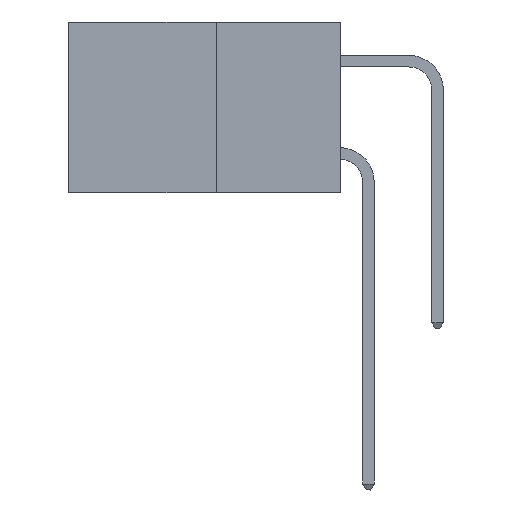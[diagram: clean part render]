
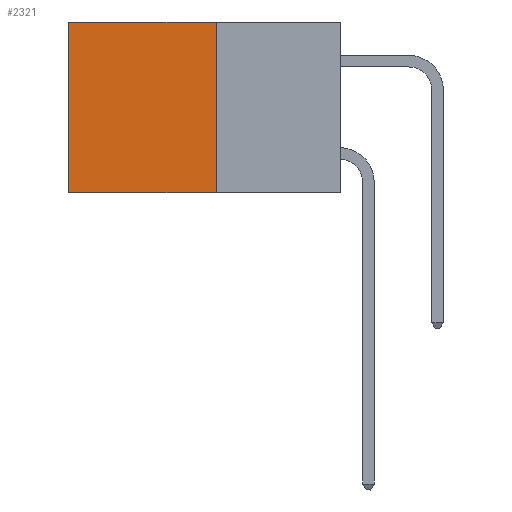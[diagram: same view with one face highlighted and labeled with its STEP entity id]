
A CAD part, left-side view. The second image highlights one B-rep face of the part: STEP entity #2321.
In plain terms, the highlighted planar face has unit normal (-1, 0, 0).
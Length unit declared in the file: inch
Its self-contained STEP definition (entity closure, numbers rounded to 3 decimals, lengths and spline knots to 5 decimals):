
#137 = ORIENTED_EDGE ( 'NONE', *, *, #2906, .F. ) ;
#462 = ORIENTED_EDGE ( 'NONE', *, *, #7147, .T. ) ;
#875 = VECTOR ( 'NONE', #17117, 39.37008 ) ;
#896 = DIRECTION ( 'NONE',  ( 0., 0., -1. ) ) ;
#1200 = CARTESIAN_POINT ( 'NONE',  ( 0.277, 0.27, -0.37 ) ) ;
#2321 = ADVANCED_FACE ( 'NONE', ( #20851 ), #13133, .F. ) ;
#2906 = EDGE_CURVE ( 'NONE', #16045, #12541, #14380, .T. ) ;
#3169 = VERTEX_POINT ( 'NONE', #16788 ) ;
#3947 = CARTESIAN_POINT ( 'NONE',  ( 0.277, 0.27, -0.37 ) ) ;
#3999 = EDGE_CURVE ( 'NONE', #3169, #19557, #19800, .T. ) ;
#6379 = ORIENTED_EDGE ( 'NONE', *, *, #10485, .F. ) ;
#7147 = EDGE_CURVE ( 'NONE', #16045, #3169, #12520, .T. ) ;
#7300 = DIRECTION ( 'NONE',  ( 0., 0., -1. ) ) ;
#7680 = ORIENTED_EDGE ( 'NONE', *, *, #3999, .T. ) ;
#7720 = CARTESIAN_POINT ( 'NONE',  ( 0.277, 0.59, -0.37 ) ) ;
#9760 = DIRECTION ( 'NONE',  ( 0., 1., 0. ) ) ;
#10485 = EDGE_CURVE ( 'NONE', #12541, #19557, #12119, .T. ) ;
#12119 = LINE ( 'NONE', #14896, #16109 ) ;
#12520 = LINE ( 'NONE', #18241, #20841 ) ;
#12541 = VERTEX_POINT ( 'NONE', #3947 ) ;
#12621 = EDGE_LOOP ( 'NONE', ( #7680, #6379, #137, #462 ) ) ;
#12766 = CARTESIAN_POINT ( 'NONE',  ( 0.277, 0.27, 0. ) ) ;
#13133 = PLANE ( 'NONE',  #13818 ) ;
#13818 = AXIS2_PLACEMENT_3D ( 'NONE', #1200, #14985, #896 ) ;
#14380 = LINE ( 'NONE', #16083, #875 ) ;
#14896 = CARTESIAN_POINT ( 'NONE',  ( 0.277, 0.27, -0.37 ) ) ;
#14985 = DIRECTION ( 'NONE',  ( 1., 0., 0. ) ) ;
#16045 = VERTEX_POINT ( 'NONE', #12766 ) ;
#16083 = CARTESIAN_POINT ( 'NONE',  ( 0.277, 0.27, -0.37 ) ) ;
#16109 = VECTOR ( 'NONE', #9760, 39.37008 ) ;
#16552 = DIRECTION ( 'NONE',  ( 0., 1., 0. ) ) ;
#16788 = CARTESIAN_POINT ( 'NONE',  ( 0.277, 0.59, 0. ) ) ;
#17117 = DIRECTION ( 'NONE',  ( 0., 0., -1. ) ) ;
#17546 = CARTESIAN_POINT ( 'NONE',  ( 0.277, 0.59, -0.37 ) ) ;
#18241 = CARTESIAN_POINT ( 'NONE',  ( 0.277, 0.27, 0. ) ) ;
#19297 = VECTOR ( 'NONE', #7300, 39.37008 ) ;
#19557 = VERTEX_POINT ( 'NONE', #17546 ) ;
#19800 = LINE ( 'NONE', #7720, #19297 ) ;
#20841 = VECTOR ( 'NONE', #16552, 39.37008 ) ;
#20851 = FACE_OUTER_BOUND ( 'NONE', #12621, .T. ) ;
